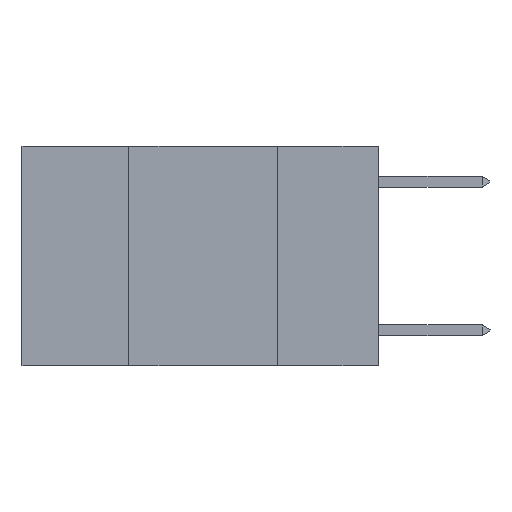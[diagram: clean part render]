
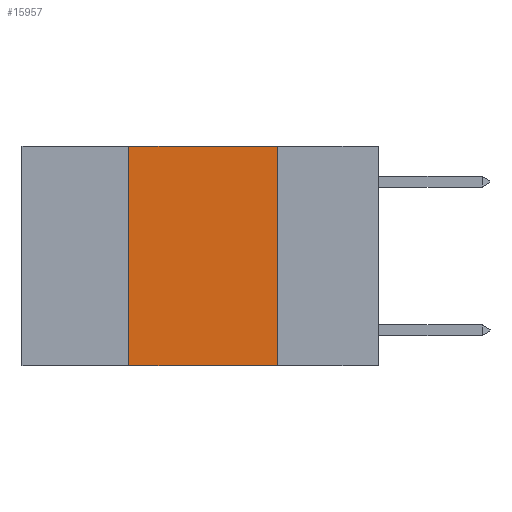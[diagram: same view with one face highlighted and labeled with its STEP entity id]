
A CAD part, left-side view. The second image highlights one B-rep face of the part: STEP entity #15957.
In plain terms, the highlighted planar face has unit normal (-1, 0, 0).
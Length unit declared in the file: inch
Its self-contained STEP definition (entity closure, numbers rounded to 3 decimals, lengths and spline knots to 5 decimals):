
#120 = CARTESIAN_POINT ( 'NONE',  ( 0., 0.6, -0.37 ) ) ;
#270 = FACE_OUTER_BOUND ( 'NONE', #7954, .T. ) ;
#1131 = LINE ( 'NONE', #9911, #14108 ) ;
#1373 = CARTESIAN_POINT ( 'NONE',  ( 0., 0.6, 0. ) ) ;
#1677 = EDGE_CURVE ( 'NONE', #8019, #3489, #5983, .T. ) ;
#2278 = VECTOR ( 'NONE', #17168, 39.37008 ) ;
#2332 = VERTEX_POINT ( 'NONE', #6926 ) ;
#2793 = DIRECTION ( 'NONE',  ( 1., 0., 0. ) ) ;
#3489 = VERTEX_POINT ( 'NONE', #13919 ) ;
#3586 = EDGE_CURVE ( 'NONE', #7238, #2332, #1131, .T. ) ;
#4433 = DIRECTION ( 'NONE',  ( 0., -1., 0. ) ) ;
#4504 = DIRECTION ( 'NONE',  ( 0., 0., -1. ) ) ;
#5191 = AXIS2_PLACEMENT_3D ( 'NONE', #1373, #2793, #12435 ) ;
#5296 = VECTOR ( 'NONE', #4433, 39.37008 ) ;
#5983 = LINE ( 'NONE', #15152, #2278 ) ;
#6926 = CARTESIAN_POINT ( 'NONE',  ( 0., 0.17, -0.37 ) ) ;
#7216 = LINE ( 'NONE', #10062, #14101 ) ;
#7238 = VERTEX_POINT ( 'NONE', #13491 ) ;
#7533 = ORIENTED_EDGE ( 'NONE', *, *, #3586, .F. ) ;
#7954 = EDGE_LOOP ( 'NONE', ( #7533, #13844, #15263, #9571 ) ) ;
#8019 = VERTEX_POINT ( 'NONE', #8148 ) ;
#8148 = CARTESIAN_POINT ( 'NONE',  ( 0., 0.42, -0.37 ) ) ;
#9367 = LINE ( 'NONE', #120, #5296 ) ;
#9571 = ORIENTED_EDGE ( 'NONE', *, *, #16729, .T. ) ;
#9697 = PLANE ( 'NONE',  #5191 ) ;
#9911 = CARTESIAN_POINT ( 'NONE',  ( 0., 0.17, 0. ) ) ;
#10062 = CARTESIAN_POINT ( 'NONE',  ( 0., 0.6, 0. ) ) ;
#11164 = EDGE_CURVE ( 'NONE', #3489, #7238, #7216, .T. ) ;
#11431 = DIRECTION ( 'NONE',  ( 0., -1., 0. ) ) ;
#12435 = DIRECTION ( 'NONE',  ( 0., 0., -1. ) ) ;
#13491 = CARTESIAN_POINT ( 'NONE',  ( 0., 0.17, 0. ) ) ;
#13844 = ORIENTED_EDGE ( 'NONE', *, *, #11164, .F. ) ;
#13919 = CARTESIAN_POINT ( 'NONE',  ( 0., 0.42, 0. ) ) ;
#14101 = VECTOR ( 'NONE', #11431, 39.37008 ) ;
#14108 = VECTOR ( 'NONE', #4504, 39.37008 ) ;
#15152 = CARTESIAN_POINT ( 'NONE',  ( 0., 0.42, 0. ) ) ;
#15263 = ORIENTED_EDGE ( 'NONE', *, *, #1677, .F. ) ;
#15957 = ADVANCED_FACE ( 'NONE', ( #270 ), #9697, .F. ) ;
#16729 = EDGE_CURVE ( 'NONE', #8019, #2332, #9367, .T. ) ;
#17168 = DIRECTION ( 'NONE',  ( 0., 0., 1. ) ) ;
